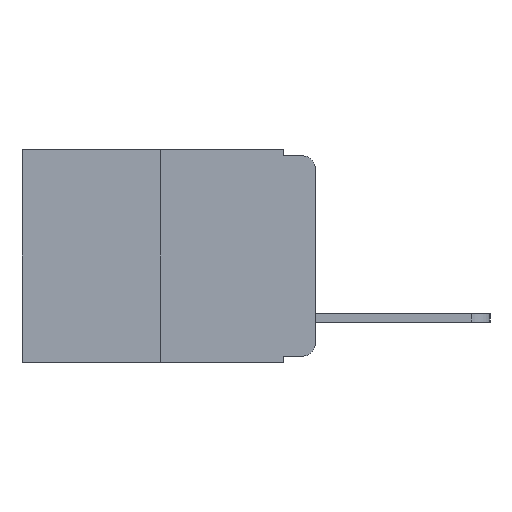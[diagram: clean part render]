
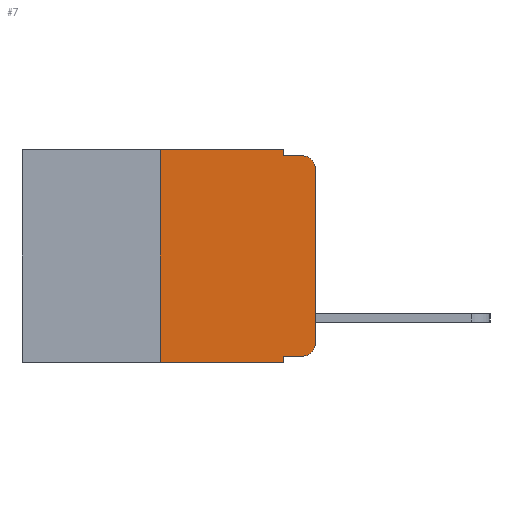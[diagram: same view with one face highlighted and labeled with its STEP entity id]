
A CAD part, left-side view. The second image highlights one B-rep face of the part: STEP entity #7.
In plain terms, the highlighted planar face has unit normal (-1, 0, 0).
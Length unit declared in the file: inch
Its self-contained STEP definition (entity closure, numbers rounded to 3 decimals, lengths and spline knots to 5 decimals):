
#7 = ADVANCED_FACE ( 'NONE', ( #8352 ), #11216, .F. ) ;
#13 = VERTEX_POINT ( 'NONE', #3124 ) ;
#35 = EDGE_CURVE ( 'NONE', #4407, #1898, #80, .T. ) ;
#80 = LINE ( 'NONE', #5978, #2970 ) ;
#108 = VERTEX_POINT ( 'NONE', #620 ) ;
#114 = CARTESIAN_POINT ( 'NONE',  ( 0., 0.02, -0.313 ) ) ;
#347 = VERTEX_POINT ( 'NONE', #9871 ) ;
#464 = VERTEX_POINT ( 'NONE', #3174 ) ;
#510 = AXIS2_PLACEMENT_3D ( 'NONE', #9676, #4176, #10535 ) ;
#620 = CARTESIAN_POINT ( 'NONE',  ( 0., 0.02, -0.01 ) ) ;
#663 = DIRECTION ( 'NONE',  ( 0., 0., -1. ) ) ;
#716 = CARTESIAN_POINT ( 'NONE',  ( 0., 0.051, 0. ) ) ;
#1017 = DIRECTION ( 'NONE',  ( 0., 0., 1. ) ) ;
#1085 = CARTESIAN_POINT ( 'NONE',  ( 0., 0.25, 0. ) ) ;
#1090 = ORIENTED_EDGE ( 'NONE', *, *, #7390, .F. ) ;
#1329 = DIRECTION ( 'NONE',  ( 0., 0., -1. ) ) ;
#1357 = DIRECTION ( 'NONE',  ( 1., 0., 0. ) ) ;
#1456 = VERTEX_POINT ( 'NONE', #6728 ) ;
#1898 = VERTEX_POINT ( 'NONE', #6479 ) ;
#2110 = CARTESIAN_POINT ( 'NONE',  ( 0., 0.25, 0. ) ) ;
#2190 = LINE ( 'NONE', #8666, #12010 ) ;
#2966 = ORIENTED_EDGE ( 'NONE', *, *, #7531, .F. ) ;
#2970 = VECTOR ( 'NONE', #3189, 39.37008 ) ;
#2973 = DIRECTION ( 'NONE',  ( 0., 0., 1. ) ) ;
#3124 = CARTESIAN_POINT ( 'NONE',  ( 0., 0.051, -0.333 ) ) ;
#3174 = CARTESIAN_POINT ( 'NONE',  ( 0., 0.051, 0. ) ) ;
#3189 = DIRECTION ( 'NONE',  ( 0., -1., 0. ) ) ;
#3242 = AXIS2_PLACEMENT_3D ( 'NONE', #5625, #1357, #11373 ) ;
#3275 = VERTEX_POINT ( 'NONE', #2110 ) ;
#3322 = VECTOR ( 'NONE', #6133, 39.37008 ) ;
#3885 = VECTOR ( 'NONE', #663, 39.37008 ) ;
#4106 = ORIENTED_EDGE ( 'NONE', *, *, #9379, .F. ) ;
#4176 = DIRECTION ( 'NONE',  ( -1., 0., 0. ) ) ;
#4226 = ORIENTED_EDGE ( 'NONE', *, *, #9918, .T. ) ;
#4345 = ORIENTED_EDGE ( 'NONE', *, *, #5071, .T. ) ;
#4407 = VERTEX_POINT ( 'NONE', #9334 ) ;
#4754 = CIRCLE ( 'NONE', #510, 0.02 ) ;
#5071 = EDGE_CURVE ( 'NONE', #13, #7526, #11772, .T. ) ;
#5099 = ORIENTED_EDGE ( 'NONE', *, *, #5686, .F. ) ;
#5107 = VECTOR ( 'NONE', #12280, 39.37008 ) ;
#5425 = LINE ( 'NONE', #8011, #9672 ) ;
#5448 = CIRCLE ( 'NONE', #11510, 0.02 ) ;
#5529 = ORIENTED_EDGE ( 'NONE', *, *, #35, .T. ) ;
#5625 = CARTESIAN_POINT ( 'NONE',  ( 0., 0.473, 0. ) ) ;
#5686 = EDGE_CURVE ( 'NONE', #13, #1898, #5425, .T. ) ;
#5978 = CARTESIAN_POINT ( 'NONE',  ( 0., 0.473, -0.343 ) ) ;
#5990 = DIRECTION ( 'NONE',  ( 0., -1., 0. ) ) ;
#6133 = DIRECTION ( 'NONE',  ( 0., -1., 0. ) ) ;
#6390 = LINE ( 'NONE', #716, #3885 ) ;
#6479 = CARTESIAN_POINT ( 'NONE',  ( 0., 0.051, -0.343 ) ) ;
#6518 = ORIENTED_EDGE ( 'NONE', *, *, #6908, .F. ) ;
#6728 = CARTESIAN_POINT ( 'NONE',  ( 0., 0., -0.313 ) ) ;
#6908 = EDGE_CURVE ( 'NONE', #4407, #3275, #11263, .T. ) ;
#6916 = DIRECTION ( 'NONE',  ( 0., 0., -1. ) ) ;
#6995 = EDGE_LOOP ( 'NONE', ( #8045, #4226, #4106, #2966, #1090, #6518, #5529, #5099, #4345, #10888 ) ) ;
#7038 = CARTESIAN_POINT ( 'NONE',  ( 0., 0.051, -0.01 ) ) ;
#7147 = DIRECTION ( 'NONE',  ( -1., 0., 0. ) ) ;
#7343 = VECTOR ( 'NONE', #5990, 39.37008 ) ;
#7390 = EDGE_CURVE ( 'NONE', #3275, #464, #12204, .T. ) ;
#7394 = CARTESIAN_POINT ( 'NONE',  ( 0., 0.051, -0.333 ) ) ;
#7526 = VERTEX_POINT ( 'NONE', #7656 ) ;
#7531 = EDGE_CURVE ( 'NONE', #464, #9473, #6390, .T. ) ;
#7598 = CARTESIAN_POINT ( 'NONE',  ( 0., 0.473, 0. ) ) ;
#7656 = CARTESIAN_POINT ( 'NONE',  ( 0., 0.02, -0.333 ) ) ;
#8011 = CARTESIAN_POINT ( 'NONE',  ( 0., 0.051, 0. ) ) ;
#8045 = ORIENTED_EDGE ( 'NONE', *, *, #10496, .T. ) ;
#8352 = FACE_OUTER_BOUND ( 'NONE', #6995, .T. ) ;
#8666 = CARTESIAN_POINT ( 'NONE',  ( 0., 0., 0. ) ) ;
#8971 = VECTOR ( 'NONE', #1017, 39.37008 ) ;
#9334 = CARTESIAN_POINT ( 'NONE',  ( 0., 0.25, -0.343 ) ) ;
#9379 = EDGE_CURVE ( 'NONE', #9473, #108, #10688, .T. ) ;
#9473 = VERTEX_POINT ( 'NONE', #11623 ) ;
#9672 = VECTOR ( 'NONE', #6916, 39.37008 ) ;
#9676 = CARTESIAN_POINT ( 'NONE',  ( 0., 0.02, -0.03 ) ) ;
#9871 = CARTESIAN_POINT ( 'NONE',  ( 0., 0., -0.03 ) ) ;
#9918 = EDGE_CURVE ( 'NONE', #347, #108, #4754, .T. ) ;
#10496 = EDGE_CURVE ( 'NONE', #1456, #347, #2190, .T. ) ;
#10535 = DIRECTION ( 'NONE',  ( 0., 0., -1. ) ) ;
#10688 = LINE ( 'NONE', #7038, #3322 ) ;
#10888 = ORIENTED_EDGE ( 'NONE', *, *, #11297, .T. ) ;
#11216 = PLANE ( 'NONE',  #3242 ) ;
#11263 = LINE ( 'NONE', #1085, #8971 ) ;
#11297 = EDGE_CURVE ( 'NONE', #7526, #1456, #5448, .T. ) ;
#11373 = DIRECTION ( 'NONE',  ( 0., 0., -1. ) ) ;
#11510 = AXIS2_PLACEMENT_3D ( 'NONE', #114, #7147, #1329 ) ;
#11623 = CARTESIAN_POINT ( 'NONE',  ( 0., 0.051, -0.01 ) ) ;
#11772 = LINE ( 'NONE', #7394, #7343 ) ;
#12010 = VECTOR ( 'NONE', #2973, 39.37008 ) ;
#12204 = LINE ( 'NONE', #7598, #5107 ) ;
#12280 = DIRECTION ( 'NONE',  ( 0., -1., 0. ) ) ;
